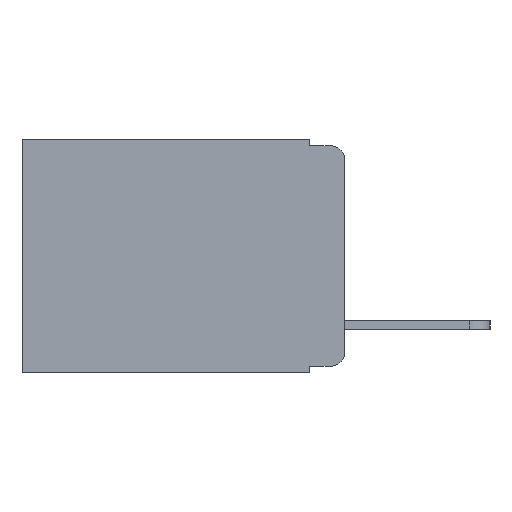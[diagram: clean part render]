
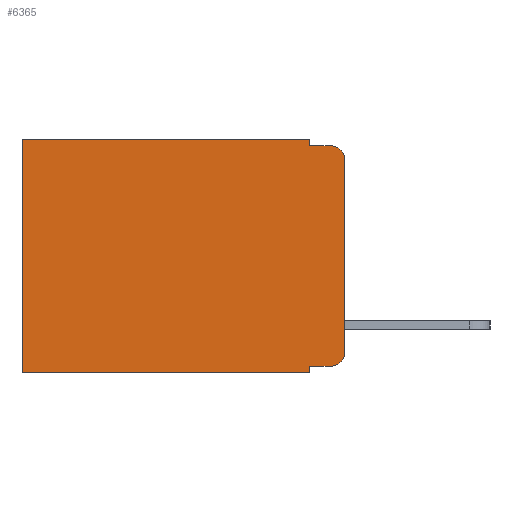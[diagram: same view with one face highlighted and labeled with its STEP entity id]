
A CAD part, left-side view. The second image highlights one B-rep face of the part: STEP entity #6365.
In plain terms, the highlighted planar face has unit normal (-1, 0, 0).
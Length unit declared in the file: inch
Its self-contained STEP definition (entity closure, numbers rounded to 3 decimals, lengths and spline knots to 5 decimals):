
#194 = LINE ( 'NONE', #9736, #9851 ) ;
#389 = VERTEX_POINT ( 'NONE', #14331 ) ;
#447 = LINE ( 'NONE', #12496, #13739 ) ;
#488 = ORIENTED_EDGE ( 'NONE', *, *, #6978, .T. ) ;
#587 = ORIENTED_EDGE ( 'NONE', *, *, #1989, .T. ) ;
#611 = VERTEX_POINT ( 'NONE', #1263 ) ;
#811 = CARTESIAN_POINT ( 'NONE',  ( 0.298, 0.02, -0.03 ) ) ;
#980 = DIRECTION ( 'NONE',  ( -1., 0., 0. ) ) ;
#1015 = EDGE_CURVE ( 'NONE', #389, #6949, #447, .T. ) ;
#1137 = VECTOR ( 'NONE', #1183, 39.37008 ) ;
#1183 = DIRECTION ( 'NONE',  ( 0., 0., -1. ) ) ;
#1263 = CARTESIAN_POINT ( 'NONE',  ( 0.298, 0.473, -0.343 ) ) ;
#1367 = VERTEX_POINT ( 'NONE', #2461 ) ;
#1465 = VECTOR ( 'NONE', #10269, 39.37008 ) ;
#1989 = EDGE_CURVE ( 'NONE', #15186, #611, #4170, .T. ) ;
#2247 = DIRECTION ( 'NONE',  ( 0., 0., -1. ) ) ;
#2461 = CARTESIAN_POINT ( 'NONE',  ( 0.298, 0.051, -0.343 ) ) ;
#2543 = LINE ( 'NONE', #6237, #12013 ) ;
#2703 = VERTEX_POINT ( 'NONE', #5206 ) ;
#2975 = VERTEX_POINT ( 'NONE', #3284 ) ;
#3284 = CARTESIAN_POINT ( 'NONE',  ( 0.298, 0.051, -0.333 ) ) ;
#3635 = AXIS2_PLACEMENT_3D ( 'NONE', #811, #16594, #16415 ) ;
#3815 = ORIENTED_EDGE ( 'NONE', *, *, #5919, .F. ) ;
#3859 = CARTESIAN_POINT ( 'NONE',  ( 0.298, 0.051, 0. ) ) ;
#3889 = CARTESIAN_POINT ( 'NONE',  ( 0.298, 0.051, 0. ) ) ;
#4032 = FACE_OUTER_BOUND ( 'NONE', #15605, .T. ) ;
#4170 = LINE ( 'NONE', #8818, #16298 ) ;
#4241 = CARTESIAN_POINT ( 'NONE',  ( 0.298, 0., -0.343 ) ) ;
#4258 = ORIENTED_EDGE ( 'NONE', *, *, #10264, .T. ) ;
#4533 = ORIENTED_EDGE ( 'NONE', *, *, #10243, .F. ) ;
#4536 = ORIENTED_EDGE ( 'NONE', *, *, #16619, .T. ) ;
#4609 = DIRECTION ( 'NONE',  ( 1., 0., 0. ) ) ;
#4706 = CARTESIAN_POINT ( 'NONE',  ( 0.298, 0.473, 0. ) ) ;
#4743 = EDGE_CURVE ( 'NONE', #1367, #611, #10561, .T. ) ;
#5206 = CARTESIAN_POINT ( 'NONE',  ( 0.298, 0.051, 0. ) ) ;
#5240 = CARTESIAN_POINT ( 'NONE',  ( 0.298, 0.02, -0.01 ) ) ;
#5398 = CIRCLE ( 'NONE', #3635, 0.02 ) ;
#5859 = VERTEX_POINT ( 'NONE', #6566 ) ;
#5870 = DIRECTION ( 'NONE',  ( 0., 1., 0. ) ) ;
#5919 = EDGE_CURVE ( 'NONE', #2703, #389, #14173, .T. ) ;
#6237 = CARTESIAN_POINT ( 'NONE',  ( 0.298, 0.051, -0.333 ) ) ;
#6365 = ADVANCED_FACE ( 'NONE', ( #4032 ), #11030, .F. ) ;
#6566 = CARTESIAN_POINT ( 'NONE',  ( 0.298, 0., -0.313 ) ) ;
#6651 = CARTESIAN_POINT ( 'NONE',  ( 0.298, 0., -0.03 ) ) ;
#6949 = VERTEX_POINT ( 'NONE', #5240 ) ;
#6978 = EDGE_CURVE ( 'NONE', #14337, #6949, #5398, .T. ) ;
#7613 = CARTESIAN_POINT ( 'NONE',  ( 0.298, 0.02, -0.333 ) ) ;
#8418 = DIRECTION ( 'NONE',  ( 0., 0., -1. ) ) ;
#8818 = CARTESIAN_POINT ( 'NONE',  ( 0.298, 0.473, 0. ) ) ;
#8864 = EDGE_CURVE ( 'NONE', #2703, #15186, #194, .T. ) ;
#9071 = DIRECTION ( 'NONE',  ( 0., -1., 0. ) ) ;
#9384 = ORIENTED_EDGE ( 'NONE', *, *, #11689, .F. ) ;
#9604 = ORIENTED_EDGE ( 'NONE', *, *, #1015, .F. ) ;
#9736 = CARTESIAN_POINT ( 'NONE',  ( 0.298, 0., 0. ) ) ;
#9851 = VECTOR ( 'NONE', #5870, 39.37008 ) ;
#9986 = LINE ( 'NONE', #3889, #1137 ) ;
#10243 = EDGE_CURVE ( 'NONE', #14337, #5859, #15454, .T. ) ;
#10264 = EDGE_CURVE ( 'NONE', #16626, #5859, #12014, .T. ) ;
#10269 = DIRECTION ( 'NONE',  ( 0., 0., -1. ) ) ;
#10561 = LINE ( 'NONE', #4241, #12756 ) ;
#10766 = DIRECTION ( 'NONE',  ( 0., 1., 0. ) ) ;
#11030 = PLANE ( 'NONE',  #14139 ) ;
#11048 = DIRECTION ( 'NONE',  ( 0., 0., -1. ) ) ;
#11084 = CARTESIAN_POINT ( 'NONE',  ( 0.298, 0., 0. ) ) ;
#11689 = EDGE_CURVE ( 'NONE', #2975, #1367, #9986, .T. ) ;
#12013 = VECTOR ( 'NONE', #9071, 39.37008 ) ;
#12014 = CIRCLE ( 'NONE', #14602, 0.02 ) ;
#12496 = CARTESIAN_POINT ( 'NONE',  ( 0.298, 0.051, -0.01 ) ) ;
#12620 = CARTESIAN_POINT ( 'NONE',  ( 0.298, 0., 0. ) ) ;
#12756 = VECTOR ( 'NONE', #10766, 39.37008 ) ;
#13044 = VECTOR ( 'NONE', #15112, 39.37008 ) ;
#13739 = VECTOR ( 'NONE', #15042, 39.37008 ) ;
#14139 = AXIS2_PLACEMENT_3D ( 'NONE', #11084, #4609, #8418 ) ;
#14173 = LINE ( 'NONE', #3859, #1465 ) ;
#14331 = CARTESIAN_POINT ( 'NONE',  ( 0.298, 0.051, -0.01 ) ) ;
#14337 = VERTEX_POINT ( 'NONE', #6651 ) ;
#14602 = AXIS2_PLACEMENT_3D ( 'NONE', #15056, #980, #2247 ) ;
#15042 = DIRECTION ( 'NONE',  ( 0., -1., 0. ) ) ;
#15056 = CARTESIAN_POINT ( 'NONE',  ( 0.298, 0.02, -0.313 ) ) ;
#15061 = ORIENTED_EDGE ( 'NONE', *, *, #8864, .T. ) ;
#15112 = DIRECTION ( 'NONE',  ( 0., 0., -1. ) ) ;
#15186 = VERTEX_POINT ( 'NONE', #4706 ) ;
#15454 = LINE ( 'NONE', #12620, #13044 ) ;
#15605 = EDGE_LOOP ( 'NONE', ( #4533, #488, #9604, #3815, #15061, #587, #16584, #9384, #4536, #4258 ) ) ;
#16298 = VECTOR ( 'NONE', #11048, 39.37008 ) ;
#16415 = DIRECTION ( 'NONE',  ( 0., 0., -1. ) ) ;
#16584 = ORIENTED_EDGE ( 'NONE', *, *, #4743, .F. ) ;
#16594 = DIRECTION ( 'NONE',  ( -1., 0., 0. ) ) ;
#16619 = EDGE_CURVE ( 'NONE', #2975, #16626, #2543, .T. ) ;
#16626 = VERTEX_POINT ( 'NONE', #7613 ) ;
